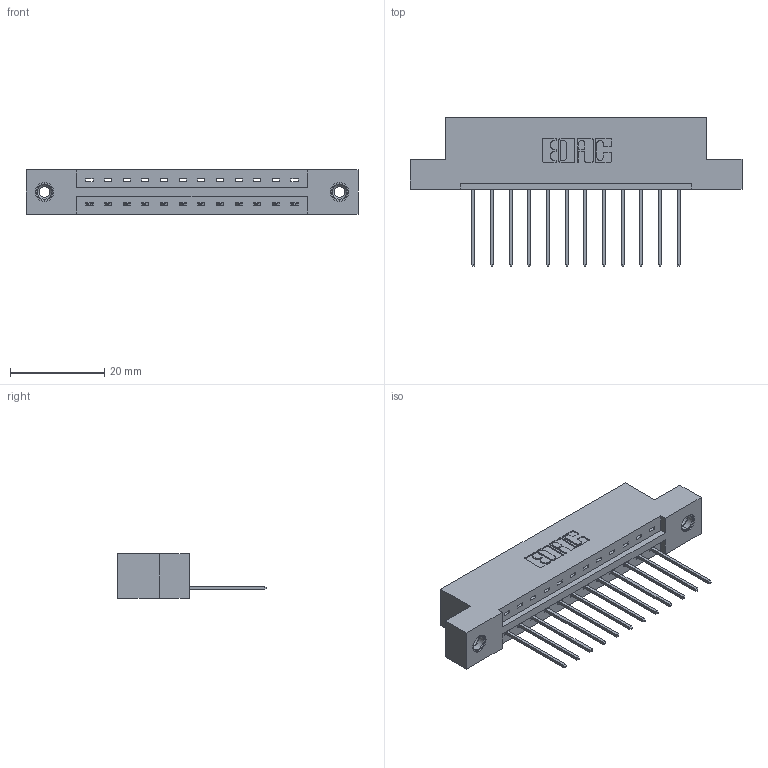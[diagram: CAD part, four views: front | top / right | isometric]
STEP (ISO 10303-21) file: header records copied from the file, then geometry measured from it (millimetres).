
FILE_DESCRIPTION (( 'STEP AP203' ), '1' );
FILE_NAME ('387-012-542-108.STEP', '2019-10-02T13:29:11', ( '' ), ( '' ), 'SwSTEP 2.0', 'SolidWorks 2016', '' );
FILE_SCHEMA (( 'CONFIG_CONTROL_DESIGN' ));
Length unit declared in the file: inch
Products named in the file (4): 345-292-001_345-293-142; 337 Part_Flush Mounting Lugs - 0.156 Dia-TI; 345-250-001_345-250-003-102; 387-012-542-108
Assembly tree (15 placements, depth 2):
  387-012-542-108
    337 Part_Flush Mounting Lugs - 0.156 Dia-TI
    345-292-001_345-293-142  x12
    345-250-001_345-250-003-102  x2
Bounding box: 70.56 x 31.63 x 9.4 mm (x, y, z)
Volume: 6978.4 mm3; surface area: 7250 mm2
Topology: 15 solids, 15 shells, 918 faces, 2703 edges, 1778 vertices
Faces by surface type: plane 654, cylinder 248, cone 12, torus 4
Entity records: 14004 total; most frequent: CARTESIAN_POINT 2417, ORIENTED_EDGE 2358, DIRECTION 2129, EDGE_CURVE 1179, VECTOR 1031, LINE 1031, VERTEX_POINT 780, AXIS2_PLACEMENT_3D 549
